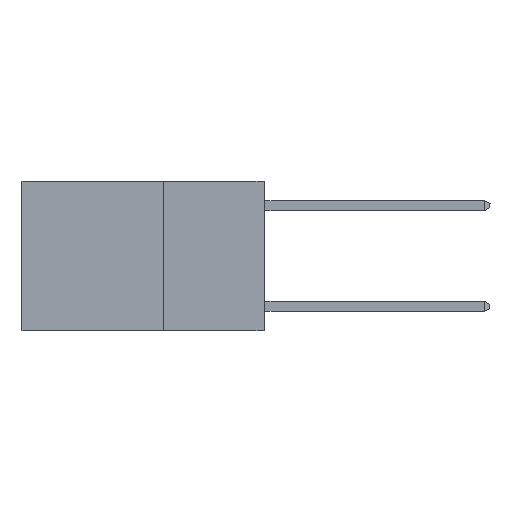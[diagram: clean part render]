
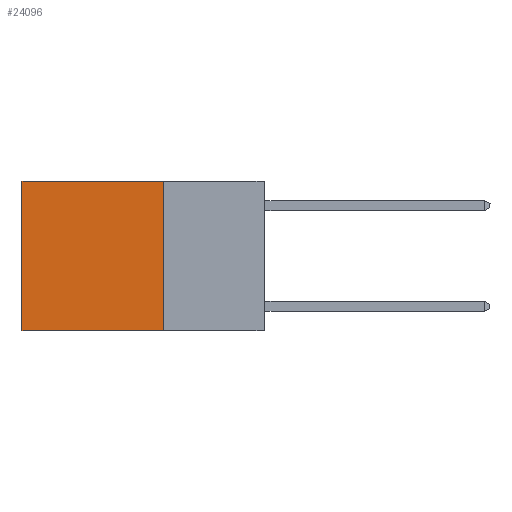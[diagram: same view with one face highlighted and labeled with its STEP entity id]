
A CAD part, left-side view. The second image highlights one B-rep face of the part: STEP entity #24096.
In plain terms, the highlighted planar face has unit normal (-1, 0, 0).
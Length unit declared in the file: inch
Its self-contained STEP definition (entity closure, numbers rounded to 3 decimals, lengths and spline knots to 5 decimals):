
#174 = ORIENTED_EDGE ( 'NONE', *, *, #11775, .T. ) ;
#288 = CARTESIAN_POINT ( 'NONE',  ( 0.2625, 0.25, 0. ) ) ;
#358 = FACE_OUTER_BOUND ( 'NONE', #2261, .T. ) ;
#779 = DIRECTION ( 'NONE',  ( 1., 0., 0. ) ) ;
#1120 = LINE ( 'NONE', #16462, #22237 ) ;
#1579 = DIRECTION ( 'NONE',  ( 0., 0., -1. ) ) ;
#1708 = VERTEX_POINT ( 'NONE', #16898 ) ;
#2051 = LINE ( 'NONE', #18049, #14066 ) ;
#2261 = EDGE_LOOP ( 'NONE', ( #174, #25607, #12539, #3883 ) ) ;
#3883 = ORIENTED_EDGE ( 'NONE', *, *, #18698, .T. ) ;
#8070 = LINE ( 'NONE', #22556, #12818 ) ;
#8770 = DIRECTION ( 'NONE',  ( 0., 1., 0. ) ) ;
#8895 = VERTEX_POINT ( 'NONE', #288 ) ;
#10431 = EDGE_CURVE ( 'NONE', #26571, #1708, #11649, .T. ) ;
#11649 = LINE ( 'NONE', #17289, #25760 ) ;
#11775 = EDGE_CURVE ( 'NONE', #16390, #1708, #8070, .T. ) ;
#11852 = EDGE_CURVE ( 'NONE', #8895, #26571, #1120, .T. ) ;
#12068 = DIRECTION ( 'NONE',  ( 0., 0., -1. ) ) ;
#12539 = ORIENTED_EDGE ( 'NONE', *, *, #11852, .F. ) ;
#12818 = VECTOR ( 'NONE', #1579, 39.37008 ) ;
#14066 = VECTOR ( 'NONE', #8770, 39.37008 ) ;
#16390 = VERTEX_POINT ( 'NONE', #22156 ) ;
#16462 = CARTESIAN_POINT ( 'NONE',  ( 0.2625, 0.25, 0. ) ) ;
#16898 = CARTESIAN_POINT ( 'NONE',  ( 0.2625, 0.6, -0.37 ) ) ;
#17289 = CARTESIAN_POINT ( 'NONE',  ( 0.2625, 0.25, -0.37 ) ) ;
#18049 = CARTESIAN_POINT ( 'NONE',  ( 0.2625, 0.25, 0. ) ) ;
#18698 = EDGE_CURVE ( 'NONE', #8895, #16390, #2051, .T. ) ;
#19287 = PLANE ( 'NONE',  #21017 ) ;
#21017 = AXIS2_PLACEMENT_3D ( 'NONE', #23980, #779, #24082 ) ;
#21052 = CARTESIAN_POINT ( 'NONE',  ( 0.2625, 0.25, -0.37 ) ) ;
#22156 = CARTESIAN_POINT ( 'NONE',  ( 0.2625, 0.6, 0. ) ) ;
#22237 = VECTOR ( 'NONE', #12068, 39.37008 ) ;
#22556 = CARTESIAN_POINT ( 'NONE',  ( 0.2625, 0.6, 0. ) ) ;
#23980 = CARTESIAN_POINT ( 'NONE',  ( 0.2625, 0.25, 0. ) ) ;
#24082 = DIRECTION ( 'NONE',  ( 0., 0., -1. ) ) ;
#24096 = ADVANCED_FACE ( 'NONE', ( #358 ), #19287, .F. ) ;
#25117 = DIRECTION ( 'NONE',  ( 0., 1., 0. ) ) ;
#25607 = ORIENTED_EDGE ( 'NONE', *, *, #10431, .F. ) ;
#25760 = VECTOR ( 'NONE', #25117, 39.37008 ) ;
#26571 = VERTEX_POINT ( 'NONE', #21052 ) ;
